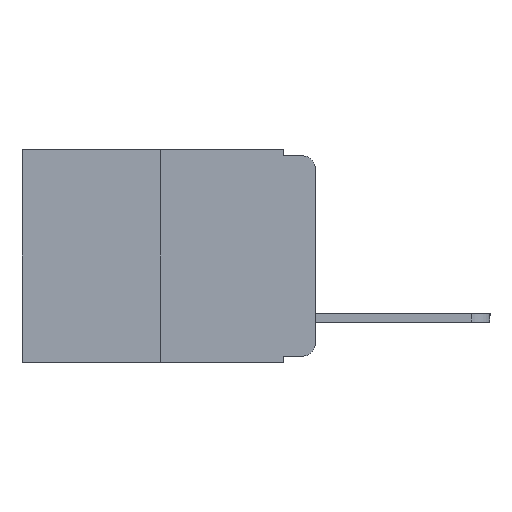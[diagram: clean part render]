
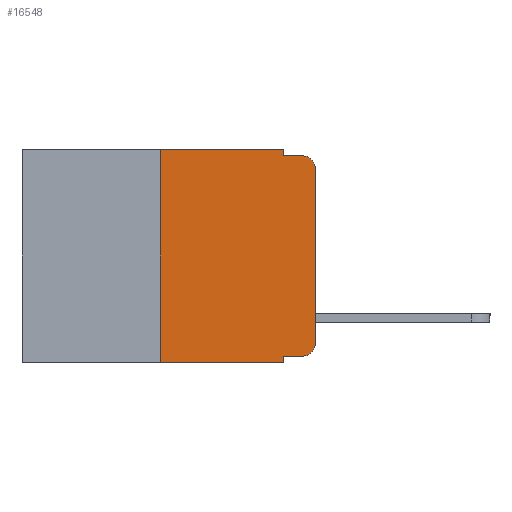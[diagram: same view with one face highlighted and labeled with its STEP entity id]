
A CAD part, left-side view. The second image highlights one B-rep face of the part: STEP entity #16548.
In plain terms, the highlighted planar face has unit normal (-1, 0, 0).
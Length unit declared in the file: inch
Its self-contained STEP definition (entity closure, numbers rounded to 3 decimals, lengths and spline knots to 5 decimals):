
#56 = DIRECTION ( 'NONE',  ( 0., 0., -1. ) ) ;
#383 = VERTEX_POINT ( 'NONE', #424 ) ;
#424 = CARTESIAN_POINT ( 'NONE',  ( 0., 0.051, -0.343 ) ) ;
#1317 = CARTESIAN_POINT ( 'NONE',  ( 0., 0.02, -0.313 ) ) ;
#1439 = DIRECTION ( 'NONE',  ( 0., -1., 0. ) ) ;
#1596 = AXIS2_PLACEMENT_3D ( 'NONE', #13363, #21547, #11806 ) ;
#1694 = CARTESIAN_POINT ( 'NONE',  ( 0., 0.051, 0. ) ) ;
#1774 = VERTEX_POINT ( 'NONE', #20436 ) ;
#2435 = VERTEX_POINT ( 'NONE', #3709 ) ;
#2527 = VECTOR ( 'NONE', #4382, 39.37008 ) ;
#3215 = DIRECTION ( 'NONE',  ( 0., 0., -1. ) ) ;
#3468 = LINE ( 'NONE', #15047, #11831 ) ;
#3709 = CARTESIAN_POINT ( 'NONE',  ( 0., 0., -0.03 ) ) ;
#3823 = CIRCLE ( 'NONE', #15715, 0.02 ) ;
#4382 = DIRECTION ( 'NONE',  ( 0., -1., 0. ) ) ;
#4393 = CARTESIAN_POINT ( 'NONE',  ( 0., 0.25, 0. ) ) ;
#4469 = ORIENTED_EDGE ( 'NONE', *, *, #6069, .T. ) ;
#5065 = CARTESIAN_POINT ( 'NONE',  ( 0., 0.473, -0.343 ) ) ;
#5562 = VERTEX_POINT ( 'NONE', #21794 ) ;
#5575 = ORIENTED_EDGE ( 'NONE', *, *, #9654, .T. ) ;
#6069 = EDGE_CURVE ( 'NONE', #17920, #383, #17066, .T. ) ;
#6183 = CARTESIAN_POINT ( 'NONE',  ( 0., 0.02, -0.333 ) ) ;
#6915 = LINE ( 'NONE', #11037, #15544 ) ;
#6932 = EDGE_CURVE ( 'NONE', #17920, #16881, #9171, .T. ) ;
#6955 = CARTESIAN_POINT ( 'NONE',  ( 0., 0.25, -0.343 ) ) ;
#7362 = DIRECTION ( 'NONE',  ( -1., 0., 0. ) ) ;
#7418 = ORIENTED_EDGE ( 'NONE', *, *, #20556, .F. ) ;
#7861 = AXIS2_PLACEMENT_3D ( 'NONE', #1317, #13211, #3215 ) ;
#8142 = EDGE_CURVE ( 'NONE', #2435, #5562, #3823, .T. ) ;
#8199 = VECTOR ( 'NONE', #16643, 39.37008 ) ;
#8434 = ORIENTED_EDGE ( 'NONE', *, *, #6932, .F. ) ;
#8924 = ORIENTED_EDGE ( 'NONE', *, *, #21793, .F. ) ;
#9171 = LINE ( 'NONE', #10232, #17316 ) ;
#9329 = CIRCLE ( 'NONE', #7861, 0.02 ) ;
#9478 = CARTESIAN_POINT ( 'NONE',  ( 0., 0., -0.313 ) ) ;
#9654 = EDGE_CURVE ( 'NONE', #10598, #18289, #9329, .T. ) ;
#10195 = ORIENTED_EDGE ( 'NONE', *, *, #13575, .T. ) ;
#10232 = CARTESIAN_POINT ( 'NONE',  ( 0., 0.25, 0. ) ) ;
#10598 = VERTEX_POINT ( 'NONE', #6183 ) ;
#11037 = CARTESIAN_POINT ( 'NONE',  ( 0., 0., 0. ) ) ;
#11487 = CARTESIAN_POINT ( 'NONE',  ( 0., 0.051, -0.333 ) ) ;
#11806 = DIRECTION ( 'NONE',  ( 0., 0., -1. ) ) ;
#11831 = VECTOR ( 'NONE', #16688, 39.37008 ) ;
#11838 = EDGE_CURVE ( 'NONE', #12043, #10598, #20717, .T. ) ;
#11880 = DIRECTION ( 'NONE',  ( 0., 0., 1. ) ) ;
#12008 = LINE ( 'NONE', #1694, #20194 ) ;
#12043 = VERTEX_POINT ( 'NONE', #11487 ) ;
#12621 = EDGE_CURVE ( 'NONE', #16881, #1774, #16846, .T. ) ;
#13211 = DIRECTION ( 'NONE',  ( -1., 0., 0. ) ) ;
#13301 = EDGE_CURVE ( 'NONE', #1774, #16265, #12008, .T. ) ;
#13363 = CARTESIAN_POINT ( 'NONE',  ( 0., 0.473, 0. ) ) ;
#13425 = CARTESIAN_POINT ( 'NONE',  ( 0., 0.473, 0. ) ) ;
#13575 = EDGE_CURVE ( 'NONE', #18289, #2435, #6915, .T. ) ;
#14244 = CARTESIAN_POINT ( 'NONE',  ( 0., 0.051, -0.333 ) ) ;
#15047 = CARTESIAN_POINT ( 'NONE',  ( 0., 0.051, -0.01 ) ) ;
#15544 = VECTOR ( 'NONE', #17608, 39.37008 ) ;
#15715 = AXIS2_PLACEMENT_3D ( 'NONE', #17092, #7362, #18775 ) ;
#16250 = LINE ( 'NONE', #20370, #19595 ) ;
#16265 = VERTEX_POINT ( 'NONE', #19244 ) ;
#16548 = ADVANCED_FACE ( 'NONE', ( #20667 ), #19975, .F. ) ;
#16560 = VECTOR ( 'NONE', #1439, 39.37008 ) ;
#16643 = DIRECTION ( 'NONE',  ( 0., -1., 0. ) ) ;
#16688 = DIRECTION ( 'NONE',  ( 0., -1., 0. ) ) ;
#16846 = LINE ( 'NONE', #13425, #8199 ) ;
#16881 = VERTEX_POINT ( 'NONE', #4393 ) ;
#17066 = LINE ( 'NONE', #5065, #16560 ) ;
#17092 = CARTESIAN_POINT ( 'NONE',  ( 0., 0.02, -0.03 ) ) ;
#17316 = VECTOR ( 'NONE', #11880, 39.37008 ) ;
#17603 = ORIENTED_EDGE ( 'NONE', *, *, #11838, .T. ) ;
#17608 = DIRECTION ( 'NONE',  ( 0., 0., 1. ) ) ;
#17920 = VERTEX_POINT ( 'NONE', #6955 ) ;
#18289 = VERTEX_POINT ( 'NONE', #9478 ) ;
#18461 = DIRECTION ( 'NONE',  ( 0., 0., -1. ) ) ;
#18775 = DIRECTION ( 'NONE',  ( 0., 0., -1. ) ) ;
#19244 = CARTESIAN_POINT ( 'NONE',  ( 0., 0.051, -0.01 ) ) ;
#19402 = ORIENTED_EDGE ( 'NONE', *, *, #8142, .T. ) ;
#19595 = VECTOR ( 'NONE', #56, 39.37008 ) ;
#19975 = PLANE ( 'NONE',  #1596 ) ;
#20194 = VECTOR ( 'NONE', #18461, 39.37008 ) ;
#20370 = CARTESIAN_POINT ( 'NONE',  ( 0., 0.051, 0. ) ) ;
#20416 = ORIENTED_EDGE ( 'NONE', *, *, #13301, .F. ) ;
#20436 = CARTESIAN_POINT ( 'NONE',  ( 0., 0.051, 0. ) ) ;
#20556 = EDGE_CURVE ( 'NONE', #16265, #5562, #3468, .T. ) ;
#20667 = FACE_OUTER_BOUND ( 'NONE', #21311, .T. ) ;
#20717 = LINE ( 'NONE', #14244, #2527 ) ;
#20910 = ORIENTED_EDGE ( 'NONE', *, *, #12621, .F. ) ;
#21311 = EDGE_LOOP ( 'NONE', ( #10195, #19402, #7418, #20416, #20910, #8434, #4469, #8924, #17603, #5575 ) ) ;
#21547 = DIRECTION ( 'NONE',  ( 1., 0., 0. ) ) ;
#21793 = EDGE_CURVE ( 'NONE', #12043, #383, #16250, .T. ) ;
#21794 = CARTESIAN_POINT ( 'NONE',  ( 0., 0.02, -0.01 ) ) ;
